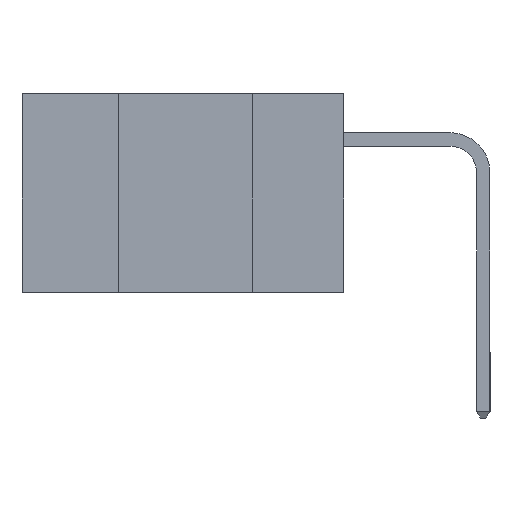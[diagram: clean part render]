
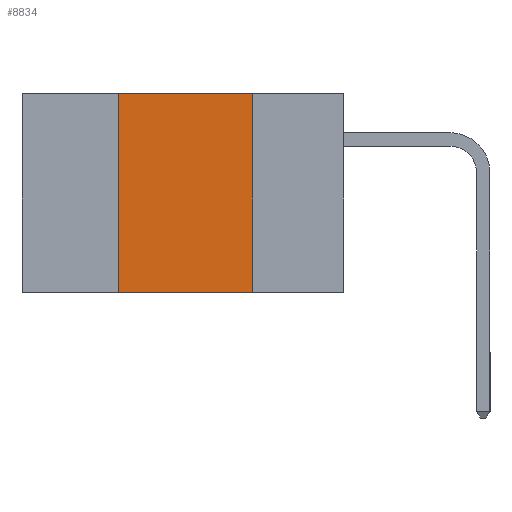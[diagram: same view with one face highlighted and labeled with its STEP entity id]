
A CAD part, left-side view. The second image highlights one B-rep face of the part: STEP entity #8834.
In plain terms, the highlighted planar face has unit normal (-1, 0, 0).
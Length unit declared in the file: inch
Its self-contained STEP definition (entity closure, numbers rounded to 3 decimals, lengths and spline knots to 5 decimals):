
#982 = VERTEX_POINT ( 'NONE', #21984 ) ;
#1518 = LINE ( 'NONE', #15877, #27534 ) ;
#3219 = LINE ( 'NONE', #5640, #26744 ) ;
#3252 = ORIENTED_EDGE ( 'NONE', *, *, #23348, .F. ) ;
#3364 = DIRECTION ( 'NONE',  ( 0., 0., -1. ) ) ;
#5531 = CARTESIAN_POINT ( 'NONE',  ( 0., 0.42, 0. ) ) ;
#5640 = CARTESIAN_POINT ( 'NONE',  ( 0., 0.6, 0. ) ) ;
#7361 = ORIENTED_EDGE ( 'NONE', *, *, #24958, .F. ) ;
#7447 = CARTESIAN_POINT ( 'NONE',  ( 0., 0.17, 0. ) ) ;
#8834 = ADVANCED_FACE ( 'NONE', ( #16577 ), #9560, .F. ) ;
#9560 = PLANE ( 'NONE',  #24594 ) ;
#9814 = VERTEX_POINT ( 'NONE', #20647 ) ;
#11440 = ORIENTED_EDGE ( 'NONE', *, *, #25843, .T. ) ;
#12606 = EDGE_CURVE ( 'NONE', #19972, #982, #22911, .T. ) ;
#12651 = CARTESIAN_POINT ( 'NONE',  ( 0., 0.17, 0. ) ) ;
#14759 = VECTOR ( 'NONE', #3364, 39.37008 ) ;
#14923 = VECTOR ( 'NONE', #22009, 39.37008 ) ;
#15358 = ORIENTED_EDGE ( 'NONE', *, *, #12606, .F. ) ;
#15877 = CARTESIAN_POINT ( 'NONE',  ( 0., 0.6, -0.37 ) ) ;
#16081 = VERTEX_POINT ( 'NONE', #22886 ) ;
#16387 = DIRECTION ( 'NONE',  ( 0., -1., 0. ) ) ;
#16577 = FACE_OUTER_BOUND ( 'NONE', #16978, .T. ) ;
#16978 = EDGE_LOOP ( 'NONE', ( #15358, #7361, #3252, #11440 ) ) ;
#19972 = VERTEX_POINT ( 'NONE', #12651 ) ;
#20647 = CARTESIAN_POINT ( 'NONE',  ( 0., 0.42, 0. ) ) ;
#21984 = CARTESIAN_POINT ( 'NONE',  ( 0., 0.17, -0.37 ) ) ;
#22009 = DIRECTION ( 'NONE',  ( 0., 0., 1. ) ) ;
#22473 = DIRECTION ( 'NONE',  ( 1., 0., 0. ) ) ;
#22886 = CARTESIAN_POINT ( 'NONE',  ( 0., 0.42, -0.37 ) ) ;
#22911 = LINE ( 'NONE', #7447, #14759 ) ;
#23348 = EDGE_CURVE ( 'NONE', #16081, #9814, #26201, .T. ) ;
#24594 = AXIS2_PLACEMENT_3D ( 'NONE', #24941, #22473, #27158 ) ;
#24939 = DIRECTION ( 'NONE',  ( 0., -1., 0. ) ) ;
#24941 = CARTESIAN_POINT ( 'NONE',  ( 0., 0.6, 0. ) ) ;
#24958 = EDGE_CURVE ( 'NONE', #9814, #19972, #3219, .T. ) ;
#25843 = EDGE_CURVE ( 'NONE', #16081, #982, #1518, .T. ) ;
#26201 = LINE ( 'NONE', #5531, #14923 ) ;
#26744 = VECTOR ( 'NONE', #16387, 39.37008 ) ;
#27158 = DIRECTION ( 'NONE',  ( 0., 0., -1. ) ) ;
#27534 = VECTOR ( 'NONE', #24939, 39.37008 ) ;
